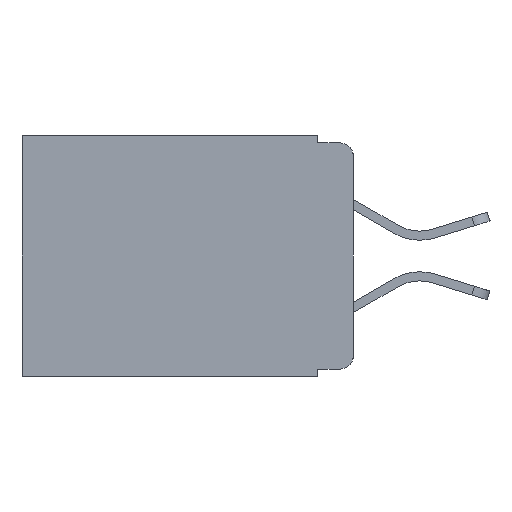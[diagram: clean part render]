
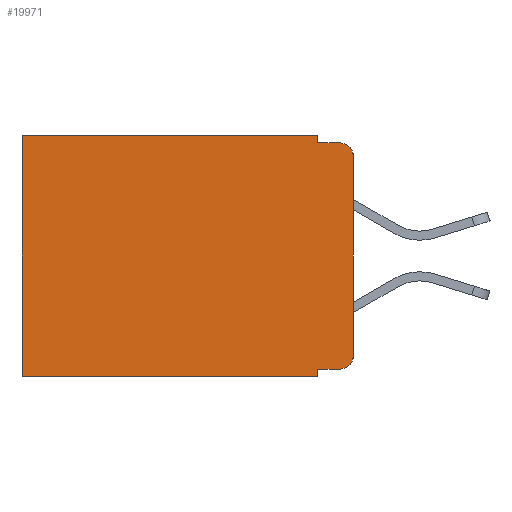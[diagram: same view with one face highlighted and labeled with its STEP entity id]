
A CAD part, left-side view. The second image highlights one B-rep face of the part: STEP entity #19971.
In plain terms, the highlighted planar face has unit normal (-1, 0, 0).
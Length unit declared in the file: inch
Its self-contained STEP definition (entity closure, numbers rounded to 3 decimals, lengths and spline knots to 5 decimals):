
#34 = VERTEX_POINT ( 'NONE', #18179 ) ;
#69 = LINE ( 'NONE', #1948, #4910 ) ;
#99 = DIRECTION ( 'NONE',  ( 0., 0., -1. ) ) ;
#196 = CARTESIAN_POINT ( 'NONE',  ( 0.298, 0., 0. ) ) ;
#890 = LINE ( 'NONE', #5886, #5165 ) ;
#1211 = VERTEX_POINT ( 'NONE', #15434 ) ;
#1236 = VERTEX_POINT ( 'NONE', #2425 ) ;
#1948 = CARTESIAN_POINT ( 'NONE',  ( 0.298, 0., -0.343 ) ) ;
#2145 = CARTESIAN_POINT ( 'NONE',  ( 0.298, 0.051, 0. ) ) ;
#2171 = VERTEX_POINT ( 'NONE', #15985 ) ;
#2203 = VERTEX_POINT ( 'NONE', #8441 ) ;
#2425 = CARTESIAN_POINT ( 'NONE',  ( 0.298, 0.051, 0. ) ) ;
#2508 = DIRECTION ( 'NONE',  ( 0., 0., -1. ) ) ;
#2862 = FACE_OUTER_BOUND ( 'NONE', #15395, .T. ) ;
#2874 = CARTESIAN_POINT ( 'NONE',  ( 0.298, 0.473, -0.343 ) ) ;
#3007 = CARTESIAN_POINT ( 'NONE',  ( 0.298, 0.051, -0.333 ) ) ;
#3291 = LINE ( 'NONE', #21651, #12524 ) ;
#3454 = DIRECTION ( 'NONE',  ( -1., 0., 0. ) ) ;
#3656 = LINE ( 'NONE', #2145, #8369 ) ;
#3971 = DIRECTION ( 'NONE',  ( 0., 0., -1. ) ) ;
#4293 = DIRECTION ( 'NONE',  ( 0., 0., -1. ) ) ;
#4363 = LINE ( 'NONE', #196, #13524 ) ;
#4392 = VECTOR ( 'NONE', #19307, 39.37008 ) ;
#4419 = DIRECTION ( 'NONE',  ( 0., 0., -1. ) ) ;
#4701 = VERTEX_POINT ( 'NONE', #8859 ) ;
#4910 = VECTOR ( 'NONE', #17415, 39.37008 ) ;
#5165 = VECTOR ( 'NONE', #7666, 39.37008 ) ;
#5265 = EDGE_CURVE ( 'NONE', #14295, #34, #20529, .T. ) ;
#5484 = LINE ( 'NONE', #13003, #14553 ) ;
#5886 = CARTESIAN_POINT ( 'NONE',  ( 0.298, 0., 0. ) ) ;
#5913 = EDGE_CURVE ( 'NONE', #2171, #34, #4363, .T. ) ;
#6116 = ORIENTED_EDGE ( 'NONE', *, *, #5265, .T. ) ;
#6248 = CARTESIAN_POINT ( 'NONE',  ( 0.298, 0.02, -0.333 ) ) ;
#6803 = ORIENTED_EDGE ( 'NONE', *, *, #19013, .T. ) ;
#7477 = EDGE_CURVE ( 'NONE', #15963, #16669, #3656, .T. ) ;
#7666 = DIRECTION ( 'NONE',  ( 0., 1., 0. ) ) ;
#7773 = AXIS2_PLACEMENT_3D ( 'NONE', #13795, #3454, #15469 ) ;
#8161 = ORIENTED_EDGE ( 'NONE', *, *, #10272, .F. ) ;
#8369 = VECTOR ( 'NONE', #3971, 39.37008 ) ;
#8441 = CARTESIAN_POINT ( 'NONE',  ( 0.298, 0.051, -0.01 ) ) ;
#8471 = PLANE ( 'NONE',  #14302 ) ;
#8552 = EDGE_CURVE ( 'NONE', #2171, #1211, #17478, .T. ) ;
#8859 = CARTESIAN_POINT ( 'NONE',  ( 0.298, 0.473, 0. ) ) ;
#9071 = EDGE_CURVE ( 'NONE', #15963, #14295, #3291, .T. ) ;
#9295 = CARTESIAN_POINT ( 'NONE',  ( 0.298, 0.02, -0.313 ) ) ;
#9350 = CARTESIAN_POINT ( 'NONE',  ( 0.298, 0.051, -0.01 ) ) ;
#9428 = EDGE_CURVE ( 'NONE', #2203, #1211, #18978, .T. ) ;
#10272 = EDGE_CURVE ( 'NONE', #1236, #2203, #5484, .T. ) ;
#11439 = ORIENTED_EDGE ( 'NONE', *, *, #7477, .F. ) ;
#11842 = DIRECTION ( 'NONE',  ( 0., 0., -1. ) ) ;
#11848 = LINE ( 'NONE', #16229, #20689 ) ;
#11961 = ORIENTED_EDGE ( 'NONE', *, *, #19727, .T. ) ;
#12524 = VECTOR ( 'NONE', #13406, 39.37008 ) ;
#13003 = CARTESIAN_POINT ( 'NONE',  ( 0.298, 0.051, 0. ) ) ;
#13406 = DIRECTION ( 'NONE',  ( 0., -1., 0. ) ) ;
#13442 = DIRECTION ( 'NONE',  ( -1., 0., 0. ) ) ;
#13524 = VECTOR ( 'NONE', #2508, 39.37008 ) ;
#13795 = CARTESIAN_POINT ( 'NONE',  ( 0.298, 0.02, -0.03 ) ) ;
#14060 = EDGE_CURVE ( 'NONE', #16669, #19887, #69, .T. ) ;
#14295 = VERTEX_POINT ( 'NONE', #6248 ) ;
#14302 = AXIS2_PLACEMENT_3D ( 'NONE', #20118, #21800, #11842 ) ;
#14553 = VECTOR ( 'NONE', #4419, 39.37008 ) ;
#15322 = CARTESIAN_POINT ( 'NONE',  ( 0.298, 0.051, -0.343 ) ) ;
#15395 = EDGE_LOOP ( 'NONE', ( #19735, #17842, #15601, #8161, #6803, #11961, #18183, #11439, #19226, #6116 ) ) ;
#15434 = CARTESIAN_POINT ( 'NONE',  ( 0.298, 0.02, -0.01 ) ) ;
#15469 = DIRECTION ( 'NONE',  ( 0., 0., -1. ) ) ;
#15601 = ORIENTED_EDGE ( 'NONE', *, *, #9428, .F. ) ;
#15963 = VERTEX_POINT ( 'NONE', #3007 ) ;
#15985 = CARTESIAN_POINT ( 'NONE',  ( 0.298, 0., -0.03 ) ) ;
#16229 = CARTESIAN_POINT ( 'NONE',  ( 0.298, 0.473, 0. ) ) ;
#16577 = AXIS2_PLACEMENT_3D ( 'NONE', #9295, #13442, #99 ) ;
#16669 = VERTEX_POINT ( 'NONE', #15322 ) ;
#17415 = DIRECTION ( 'NONE',  ( 0., 1., 0. ) ) ;
#17478 = CIRCLE ( 'NONE', #7773, 0.02 ) ;
#17842 = ORIENTED_EDGE ( 'NONE', *, *, #8552, .T. ) ;
#18179 = CARTESIAN_POINT ( 'NONE',  ( 0.298, 0., -0.313 ) ) ;
#18183 = ORIENTED_EDGE ( 'NONE', *, *, #14060, .F. ) ;
#18978 = LINE ( 'NONE', #9350, #4392 ) ;
#19013 = EDGE_CURVE ( 'NONE', #1236, #4701, #890, .T. ) ;
#19226 = ORIENTED_EDGE ( 'NONE', *, *, #9071, .T. ) ;
#19307 = DIRECTION ( 'NONE',  ( 0., -1., 0. ) ) ;
#19727 = EDGE_CURVE ( 'NONE', #4701, #19887, #11848, .T. ) ;
#19735 = ORIENTED_EDGE ( 'NONE', *, *, #5913, .F. ) ;
#19887 = VERTEX_POINT ( 'NONE', #2874 ) ;
#19971 = ADVANCED_FACE ( 'NONE', ( #2862 ), #8471, .F. ) ;
#20118 = CARTESIAN_POINT ( 'NONE',  ( 0.298, 0., 0. ) ) ;
#20529 = CIRCLE ( 'NONE', #16577, 0.02 ) ;
#20689 = VECTOR ( 'NONE', #4293, 39.37008 ) ;
#21651 = CARTESIAN_POINT ( 'NONE',  ( 0.298, 0.051, -0.333 ) ) ;
#21800 = DIRECTION ( 'NONE',  ( 1., 0., 0. ) ) ;
